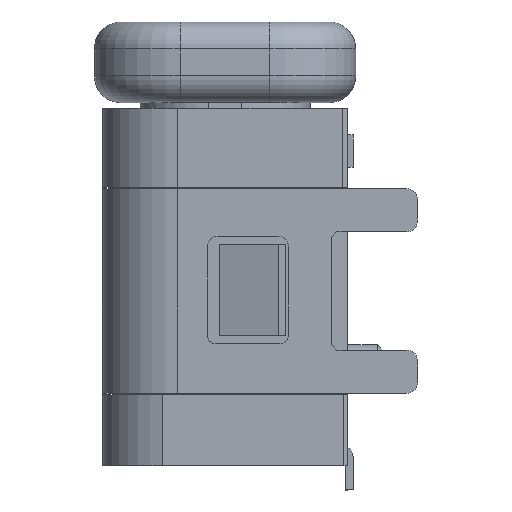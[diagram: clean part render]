
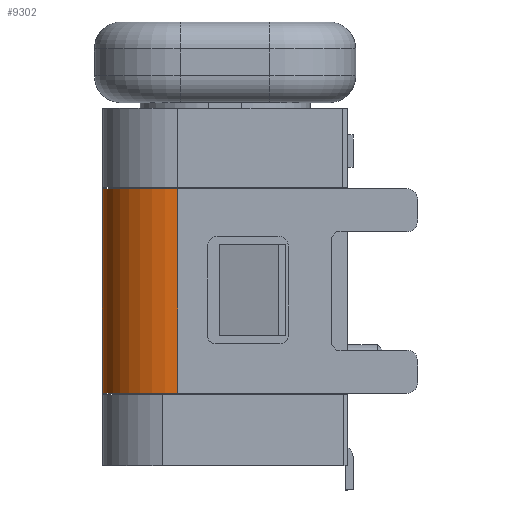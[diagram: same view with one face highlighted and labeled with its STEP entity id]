
A CAD part, left-side view. The second image highlights one B-rep face of the part: STEP entity #9302.
In plain terms, the highlighted cylindrical face has radius 1.4 mm (diameter 2.8 mm), a partial arc.
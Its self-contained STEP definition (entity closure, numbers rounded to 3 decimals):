
#690 = VERTEX_POINT ( 'NONE', #10855 ) ;
#957 = ORIENTED_EDGE ( 'NONE', *, *, #18261, .F. ) ;
#995 = LINE ( 'NONE', #20093, #5263 ) ;
#1178 = DIRECTION ( 'NONE',  ( 1., 0., 0. ) ) ;
#1307 = AXIS2_PLACEMENT_3D ( 'NONE', #13988, #14091, #19139 ) ;
#2301 = CARTESIAN_POINT ( 'NONE',  ( 3.6, 0.875, -20.941 ) ) ;
#3034 = LINE ( 'NONE', #6830, #14238 ) ;
#4427 = DIRECTION ( 'NONE',  ( 0., 0., 1. ) ) ;
#4994 = CARTESIAN_POINT ( 'NONE',  ( 5., 0.875, -8.008 ) ) ;
#5263 = VECTOR ( 'NONE', #14819, 1000. ) ;
#5310 = VERTEX_POINT ( 'NONE', #4994 ) ;
#5746 = EDGE_CURVE ( 'NONE', #690, #7274, #18086, .T. ) ;
#6815 = EDGE_CURVE ( 'NONE', #5310, #10516, #19679, .T. ) ;
#6830 = CARTESIAN_POINT ( 'NONE',  ( 5., 0.875, -9.508 ) ) ;
#7274 = VERTEX_POINT ( 'NONE', #14179 ) ;
#9302 = ADVANCED_FACE ( 'NONE', ( #19084 ), #19508, .T. ) ;
#10030 = AXIS2_PLACEMENT_3D ( 'NONE', #19746, #4427, #1178 ) ;
#10516 = VERTEX_POINT ( 'NONE', #16058 ) ;
#10855 = CARTESIAN_POINT ( 'NONE',  ( 3.6, 2.275, -4.208 ) ) ;
#11473 = ORIENTED_EDGE ( 'NONE', *, *, #6815, .T. ) ;
#11848 = ORIENTED_EDGE ( 'NONE', *, *, #5746, .T. ) ;
#12804 = EDGE_CURVE ( 'NONE', #10516, #690, #995, .T. ) ;
#13652 = DIRECTION ( 'NONE',  ( 0., 0., 1. ) ) ;
#13988 = CARTESIAN_POINT ( 'NONE',  ( 3.6, 0.875, -4.208 ) ) ;
#14091 = DIRECTION ( 'NONE',  ( 0., 0., -1. ) ) ;
#14179 = CARTESIAN_POINT ( 'NONE',  ( 5., 0.875, -4.208 ) ) ;
#14238 = VECTOR ( 'NONE', #13652, 1000. ) ;
#14819 = DIRECTION ( 'NONE',  ( 0., 0., 1. ) ) ;
#15991 = AXIS2_PLACEMENT_3D ( 'NONE', #2301, #17706, #16032 ) ;
#16032 = DIRECTION ( 'NONE',  ( 1., 0., 0. ) ) ;
#16058 = CARTESIAN_POINT ( 'NONE',  ( 3.6, 2.275, -8.008 ) ) ;
#16544 = EDGE_LOOP ( 'NONE', ( #20304, #11848, #957, #11473 ) ) ;
#17706 = DIRECTION ( 'NONE',  ( 0., 0., 1. ) ) ;
#18086 = CIRCLE ( 'NONE', #1307, 1.4 ) ;
#18261 = EDGE_CURVE ( 'NONE', #5310, #7274, #3034, .T. ) ;
#19084 = FACE_OUTER_BOUND ( 'NONE', #16544, .T. ) ;
#19139 = DIRECTION ( 'NONE',  ( 1., 0., 0. ) ) ;
#19508 = CYLINDRICAL_SURFACE ( 'NONE', #15991, 1.4 ) ;
#19679 = CIRCLE ( 'NONE', #10030, 1.4 ) ;
#19746 = CARTESIAN_POINT ( 'NONE',  ( 3.6, 0.875, -8.008 ) ) ;
#20093 = CARTESIAN_POINT ( 'NONE',  ( 3.6, 2.275, -20.941 ) ) ;
#20304 = ORIENTED_EDGE ( 'NONE', *, *, #12804, .T. ) ;
